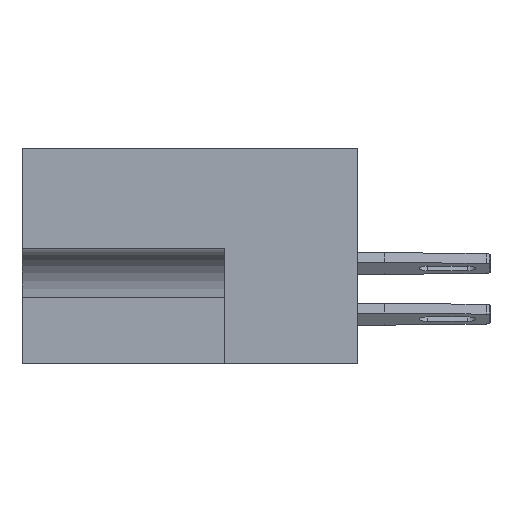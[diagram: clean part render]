
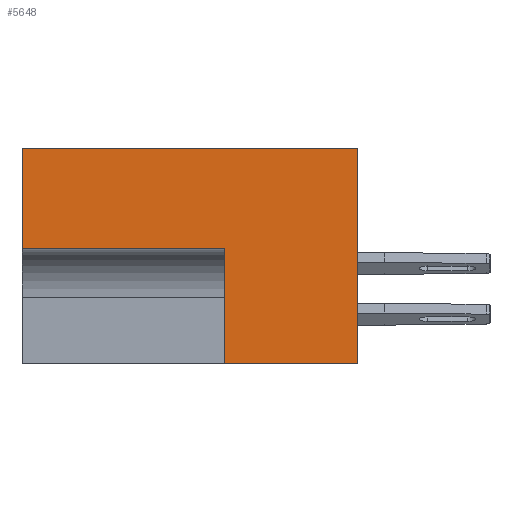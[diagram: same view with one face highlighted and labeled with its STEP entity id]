
A CAD part, left-side view. The second image highlights one B-rep face of the part: STEP entity #5648.
In plain terms, the highlighted planar face has unit normal (-1, 0, 0).
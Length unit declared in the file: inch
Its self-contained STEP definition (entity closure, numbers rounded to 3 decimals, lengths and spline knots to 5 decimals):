
#722 = LINE ( 'NONE', #13918, #7867 ) ;
#1469 = EDGE_CURVE ( 'NONE', #18410, #17137, #722, .T. ) ;
#1705 = DIRECTION ( 'NONE',  ( 0., 0., 1. ) ) ;
#1790 = VERTEX_POINT ( 'NONE', #18315 ) ;
#2192 = ORIENTED_EDGE ( 'NONE', *, *, #12202, .T. ) ;
#2508 = CARTESIAN_POINT ( 'NONE',  ( 0., 0., -0.531 ) ) ;
#2515 = VECTOR ( 'NONE', #1705, 39.37008 ) ;
#2968 = FACE_OUTER_BOUND ( 'NONE', #14700, .T. ) ;
#3180 = LINE ( 'NONE', #16711, #19710 ) ;
#3501 = VERTEX_POINT ( 'NONE', #18913 ) ;
#4155 = CARTESIAN_POINT ( 'NONE',  ( 0., 0.453, -0.531 ) ) ;
#4202 = CARTESIAN_POINT ( 'NONE',  ( 0., 0.328, -0.531 ) ) ;
#4880 = AXIS2_PLACEMENT_3D ( 'NONE', #6635, #17204, #11034 ) ;
#5234 = EDGE_CURVE ( 'NONE', #8701, #18410, #9930, .T. ) ;
#5648 = ADVANCED_FACE ( 'NONE', ( #2968 ), #8136, .F. ) ;
#6076 = CARTESIAN_POINT ( 'NONE',  ( 0., 0.453, 0. ) ) ;
#6199 = EDGE_CURVE ( 'NONE', #10895, #3501, #3180, .T. ) ;
#6635 = CARTESIAN_POINT ( 'NONE',  ( 0., 0.453, 0. ) ) ;
#7851 = VECTOR ( 'NONE', #10466, 39.37008 ) ;
#7867 = VECTOR ( 'NONE', #13850, 39.37008 ) ;
#8085 = VECTOR ( 'NONE', #9808, 39.37008 ) ;
#8136 = PLANE ( 'NONE',  #4880 ) ;
#8222 = VECTOR ( 'NONE', #8569, 39.37008 ) ;
#8569 = DIRECTION ( 'NONE',  ( 0., -1., 0. ) ) ;
#8701 = VERTEX_POINT ( 'NONE', #4202 ) ;
#9345 = CARTESIAN_POINT ( 'NONE',  ( 0., 0.328, -0.248 ) ) ;
#9808 = DIRECTION ( 'NONE',  ( 0., 0., 1. ) ) ;
#9930 = LINE ( 'NONE', #13903, #2515 ) ;
#10394 = LINE ( 'NONE', #4155, #8222 ) ;
#10412 = ORIENTED_EDGE ( 'NONE', *, *, #5234, .F. ) ;
#10466 = DIRECTION ( 'NONE',  ( 0., -1., 0. ) ) ;
#10612 = ORIENTED_EDGE ( 'NONE', *, *, #1469, .F. ) ;
#10895 = VERTEX_POINT ( 'NONE', #2508 ) ;
#11034 = DIRECTION ( 'NONE',  ( 0., 0., -1. ) ) ;
#11945 = LINE ( 'NONE', #6076, #7851 ) ;
#12202 = EDGE_CURVE ( 'NONE', #8701, #10895, #10394, .T. ) ;
#13850 = DIRECTION ( 'NONE',  ( 0., 1., 0. ) ) ;
#13903 = CARTESIAN_POINT ( 'NONE',  ( 0., 0.328, -0.531 ) ) ;
#13918 = CARTESIAN_POINT ( 'NONE',  ( 0., 0.328, -0.248 ) ) ;
#14510 = CARTESIAN_POINT ( 'NONE',  ( 0., 0.828, 0. ) ) ;
#14700 = EDGE_LOOP ( 'NONE', ( #19652, #10612, #10412, #2192, #15090, #16346 ) ) ;
#15090 = ORIENTED_EDGE ( 'NONE', *, *, #6199, .T. ) ;
#16346 = ORIENTED_EDGE ( 'NONE', *, *, #18883, .F. ) ;
#16711 = CARTESIAN_POINT ( 'NONE',  ( 0., 0., 0. ) ) ;
#16897 = DIRECTION ( 'NONE',  ( 0., 0., 1. ) ) ;
#17137 = VERTEX_POINT ( 'NONE', #17915 ) ;
#17204 = DIRECTION ( 'NONE',  ( 1., 0., 0. ) ) ;
#17231 = LINE ( 'NONE', #14510, #8085 ) ;
#17915 = CARTESIAN_POINT ( 'NONE',  ( 0., 0.828, -0.248 ) ) ;
#18315 = CARTESIAN_POINT ( 'NONE',  ( 0., 0.828, 0. ) ) ;
#18410 = VERTEX_POINT ( 'NONE', #9345 ) ;
#18638 = EDGE_CURVE ( 'NONE', #17137, #1790, #17231, .T. ) ;
#18883 = EDGE_CURVE ( 'NONE', #1790, #3501, #11945, .T. ) ;
#18913 = CARTESIAN_POINT ( 'NONE',  ( 0., 0., 0. ) ) ;
#19652 = ORIENTED_EDGE ( 'NONE', *, *, #18638, .F. ) ;
#19710 = VECTOR ( 'NONE', #16897, 39.37008 ) ;
